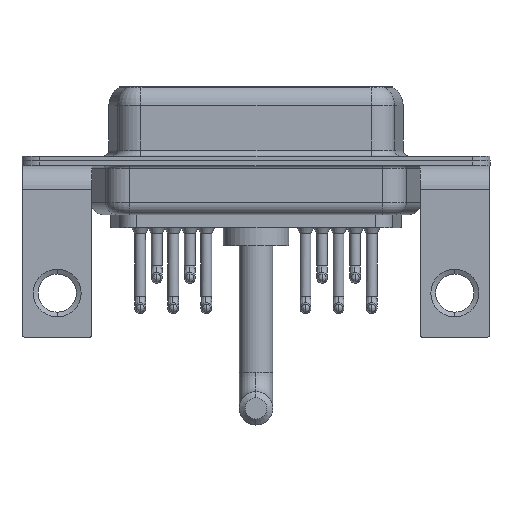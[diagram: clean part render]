
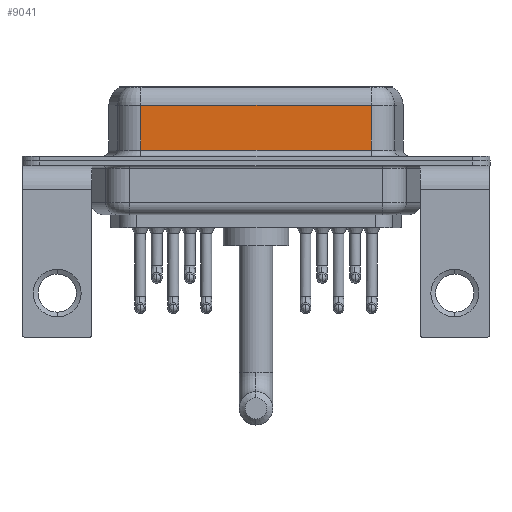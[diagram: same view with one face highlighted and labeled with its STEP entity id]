
A CAD part, front view. The second image highlights one B-rep face of the part: STEP entity #9041.
In plain terms, the highlighted planar face has unit normal (0, -1, 0).
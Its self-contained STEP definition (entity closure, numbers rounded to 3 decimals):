
#1491 = LINE ( 'NONE', #13037, #15029 ) ;
#1567 = DIRECTION ( 'NONE',  ( 0., 0., -1. ) ) ;
#2111 = EDGE_LOOP ( 'NONE', ( #5905, #14676, #10881, #4731 ) ) ;
#2474 = DIRECTION ( 'NONE',  ( 0., 0., 1. ) ) ;
#3161 = VECTOR ( 'NONE', #15467, 1000. ) ;
#4087 = EDGE_CURVE ( 'NONE', #12411, #14629, #18418, .T. ) ;
#4731 = ORIENTED_EDGE ( 'NONE', *, *, #11484, .T. ) ;
#5137 = DIRECTION ( 'NONE',  ( 0., 1., 0. ) ) ;
#5282 = CARTESIAN_POINT ( 'NONE',  ( 26.287, -3.95, 0.9 ) ) ;
#5905 = ORIENTED_EDGE ( 'NONE', *, *, #17459, .F. ) ;
#6306 = CARTESIAN_POINT ( 'NONE',  ( 7.013, -3.95, 0.9 ) ) ;
#7472 = DIRECTION ( 'NONE',  ( 0., 0., -1. ) ) ;
#8215 = VERTEX_POINT ( 'NONE', #18041 ) ;
#8378 = PLANE ( 'NONE',  #10329 ) ;
#8573 = FACE_OUTER_BOUND ( 'NONE', #2111, .T. ) ;
#9041 = ADVANCED_FACE ( 'NONE', ( #8573 ), #8378, .F. ) ;
#9678 = VECTOR ( 'NONE', #1567, 1000. ) ;
#10207 = CARTESIAN_POINT ( 'NONE',  ( 7.013, -3.95, 4.65 ) ) ;
#10329 = AXIS2_PLACEMENT_3D ( 'NONE', #18650, #5137, #2474 ) ;
#10881 = ORIENTED_EDGE ( 'NONE', *, *, #16986, .T. ) ;
#11389 = LINE ( 'NONE', #5282, #14900 ) ;
#11484 = EDGE_CURVE ( 'NONE', #18377, #8215, #11389, .T. ) ;
#12411 = VERTEX_POINT ( 'NONE', #17238 ) ;
#12693 = DIRECTION ( 'NONE',  ( 1., 0., 0. ) ) ;
#13037 = CARTESIAN_POINT ( 'NONE',  ( 7.013, -3.95, 6.4 ) ) ;
#13285 = CARTESIAN_POINT ( 'NONE',  ( 26.287, -3.95, 6.4 ) ) ;
#13679 = LINE ( 'NONE', #13285, #9678 ) ;
#14629 = VERTEX_POINT ( 'NONE', #10207 ) ;
#14676 = ORIENTED_EDGE ( 'NONE', *, *, #4087, .T. ) ;
#14900 = VECTOR ( 'NONE', #12693, 1000. ) ;
#15029 = VECTOR ( 'NONE', #7472, 1000. ) ;
#15467 = DIRECTION ( 'NONE',  ( -1., 0., 0. ) ) ;
#15659 = CARTESIAN_POINT ( 'NONE',  ( 26.287, -3.95, 4.65 ) ) ;
#16986 = EDGE_CURVE ( 'NONE', #14629, #18377, #1491, .T. ) ;
#17238 = CARTESIAN_POINT ( 'NONE',  ( 26.287, -3.95, 4.65 ) ) ;
#17459 = EDGE_CURVE ( 'NONE', #12411, #8215, #13679, .T. ) ;
#18041 = CARTESIAN_POINT ( 'NONE',  ( 26.287, -3.95, 0.9 ) ) ;
#18377 = VERTEX_POINT ( 'NONE', #6306 ) ;
#18418 = LINE ( 'NONE', #15659, #3161 ) ;
#18650 = CARTESIAN_POINT ( 'NONE',  ( 26.287, -3.95, 6.4 ) ) ;
